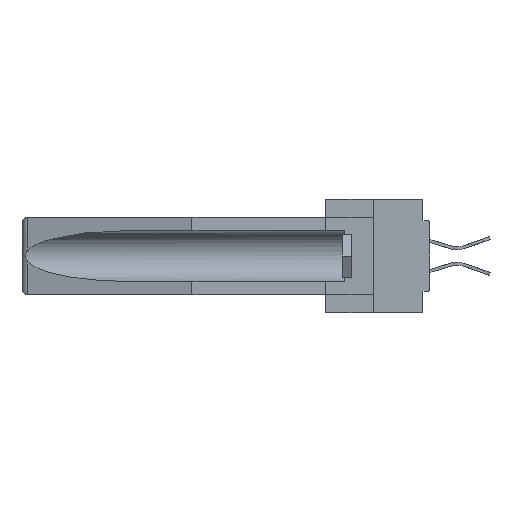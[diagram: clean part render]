
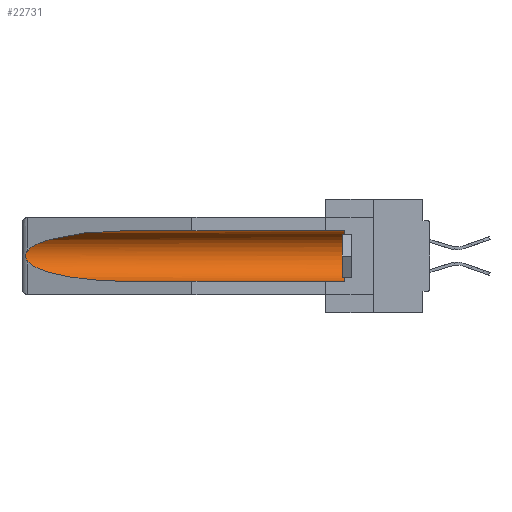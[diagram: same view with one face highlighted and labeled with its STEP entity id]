
A CAD part, left-side view. The second image highlights one B-rep face of the part: STEP entity #22731.
In plain terms, the highlighted cylindrical face has radius 2.857 mm (diameter 5.715 mm), a partial arc.
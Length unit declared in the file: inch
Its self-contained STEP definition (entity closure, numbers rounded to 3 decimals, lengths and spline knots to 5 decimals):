
#87 = DIRECTION ( 'NONE',  ( 0., 1., 0. ) ) ;
#772 = CARTESIAN_POINT ( 'NONE',  ( 0.155, 0.126, -0.1715 ) ) ;
#1857 =( BOUNDED_CURVE ( )  B_SPLINE_CURVE ( 3, ( #37850, #8240, #2736, #37587 ),
 .UNSPECIFIED., .F., .F. ) 
 B_SPLINE_CURVE_WITH_KNOTS ( ( 4, 4 ),
 ( 0.1948, 1.5708 ),
 .UNSPECIFIED. ) 
 CURVE ( )  GEOMETRIC_REPRESENTATION_ITEM ( )  RATIONAL_B_SPLINE_CURVE ( ( 1., 0.848, 0.848, 1. ) ) 
 REPRESENTATION_ITEM ( '' )  );
#2736 = CARTESIAN_POINT ( 'NONE',  ( 0.21114, 1.30732, -0.284 ) ) ;
#4269 = CARTESIAN_POINT ( 'NONE',  ( 0.26597, 1.5296, -0.19026 ) ) ;
#4793 = EDGE_CURVE ( 'NONE', #7415, #30920, #1857, .T. ) ;
#5750 = CARTESIAN_POINT ( 'NONE',  ( 0.155, -0.30754, -0.059 ) ) ;
#6039 = ORIENTED_EDGE ( 'NONE', *, *, #6914, .T. ) ;
#6296 = DIRECTION ( 'NONE',  ( 0., 1., 0. ) ) ;
#6306 = ORIENTED_EDGE ( 'NONE', *, *, #4793, .T. ) ;
#6914 = EDGE_CURVE ( 'NONE', #28909, #23332, #20168, .T. ) ;
#6995 = ORIENTED_EDGE ( 'NONE', *, *, #14055, .T. ) ;
#7080 = CARTESIAN_POINT ( 'NONE',  ( 0.2675, 1.53308, -0.17534 ) ) ;
#7415 = VERTEX_POINT ( 'NONE', #16191 ) ;
#8240 = CARTESIAN_POINT ( 'NONE',  ( 0.25451, 1.48313, -0.24835 ) ) ;
#8750 = CARTESIAN_POINT ( 'NONE',  ( 0.155, 1.07973, -0.284 ) ) ;
#9074 = CARTESIAN_POINT ( 'NONE',  ( 0.155, -0.30754, -0.284 ) ) ;
#9399 = CARTESIAN_POINT ( 'NONE',  ( 0.26654, 1.53092, -0.15636 ) ) ;
#10024 = CARTESIAN_POINT ( 'NONE',  ( 0.26537, 1.52718, -0.19328 ) ) ;
#10286 = FACE_OUTER_BOUND ( 'NONE', #32489, .T. ) ;
#10372 = CARTESIAN_POINT ( 'NONE',  ( 0.155, 1.07973, -0.059 ) ) ;
#10424 = CARTESIAN_POINT ( 'NONE',  ( 0.2673, 1.5327, -0.16383 ) ) ;
#10641 = CARTESIAN_POINT ( 'NONE',  ( 0.155, 1.07973, -0.059 ) ) ;
#11722 = AXIS2_PLACEMENT_3D ( 'NONE', #772, #21275, #12678 ) ;
#12678 = DIRECTION ( 'NONE',  ( 0., 0., 1. ) ) ;
#14055 = EDGE_CURVE ( 'NONE', #23332, #7415, #35924, .T. ) ;
#15910 = CARTESIAN_POINT ( 'NONE',  ( 0.26655, 1.53094, -0.18657 ) ) ;
#16191 = CARTESIAN_POINT ( 'NONE',  ( 0.26537, 1.52718, -0.19328 ) ) ;
#19042 = LINE ( 'NONE', #9074, #26849 ) ;
#19196 = CARTESIAN_POINT ( 'NONE',  ( 0.25451, 1.48313, -0.09465 ) ) ;
#19502 = EDGE_CURVE ( 'NONE', #28320, #19665, #35521, .T. ) ;
#19665 = VERTEX_POINT ( 'NONE', #27777 ) ;
#20168 =( BOUNDED_CURVE ( )  B_SPLINE_CURVE ( 3, ( #10372, #33806, #19196, #22140 ),
 .UNSPECIFIED., .F., .F. ) 
 B_SPLINE_CURVE_WITH_KNOTS ( ( 4, 4 ),
 ( 4.71239, 6.08839 ),
 .UNSPECIFIED. ) 
 CURVE ( )  GEOMETRIC_REPRESENTATION_ITEM ( )  RATIONAL_B_SPLINE_CURVE ( ( 1., 0.848, 0.848, 1. ) ) 
 REPRESENTATION_ITEM ( '' )  );
#21275 = DIRECTION ( 'NONE',  ( 0., -1., 0. ) ) ;
#22140 = CARTESIAN_POINT ( 'NONE',  ( 0.26537, 1.52718, -0.14972 ) ) ;
#22731 = ADVANCED_FACE ( 'NONE', ( #10286 ), #35518, .F. ) ;
#23332 = VERTEX_POINT ( 'NONE', #31109 ) ;
#23337 = ORIENTED_EDGE ( 'NONE', *, *, #19502, .T. ) ;
#23978 = CARTESIAN_POINT ( 'NONE',  ( 0.26597, 1.52961, -0.15275 ) ) ;
#26774 = CARTESIAN_POINT ( 'NONE',  ( 0.155, -0.30754, -0.1715 ) ) ;
#26849 = VECTOR ( 'NONE', #87, 39.37008 ) ;
#27563 = CARTESIAN_POINT ( 'NONE',  ( 0.2673, 1.53269, -0.17917 ) ) ;
#27777 = CARTESIAN_POINT ( 'NONE',  ( 0.155, 0.126, -0.059 ) ) ;
#28288 = CARTESIAN_POINT ( 'NONE',  ( 0.155, 0.126, -0.284 ) ) ;
#28320 = VERTEX_POINT ( 'NONE', #28288 ) ;
#28909 = VERTEX_POINT ( 'NONE', #10641 ) ;
#29865 = CARTESIAN_POINT ( 'NONE',  ( 0.2675, 1.53308, -0.16763 ) ) ;
#30920 = VERTEX_POINT ( 'NONE', #8750 ) ;
#31109 = CARTESIAN_POINT ( 'NONE',  ( 0.26537, 1.52718, -0.14972 ) ) ;
#31527 = EDGE_CURVE ( 'NONE', #19665, #28909, #34534, .T. ) ;
#32489 = EDGE_LOOP ( 'NONE', ( #6039, #6995, #6306, #33144, #23337, #37250 ) ) ;
#32511 = DIRECTION ( 'NONE',  ( 0., 1., 0. ) ) ;
#33144 = ORIENTED_EDGE ( 'NONE', *, *, #36436, .F. ) ;
#33579 = VECTOR ( 'NONE', #32511, 39.37008 ) ;
#33806 = CARTESIAN_POINT ( 'NONE',  ( 0.21114, 1.30732, -0.059 ) ) ;
#34534 = LINE ( 'NONE', #5750, #33579 ) ;
#35518 = CYLINDRICAL_SURFACE ( 'NONE', #35853, 0.1125 ) ;
#35521 = CIRCLE ( 'NONE', #11722, 0.1125 ) ;
#35853 = AXIS2_PLACEMENT_3D ( 'NONE', #26774, #6296, #35863 ) ;
#35863 = DIRECTION ( 'NONE',  ( 0., 0., 1. ) ) ;
#35924 = B_SPLINE_CURVE_WITH_KNOTS ( 'NONE', 3,
 ( #36421, #23978, #9399, #10424, #29865, #7080, #27563, #15910, #4269, #10024 ),
 .UNSPECIFIED., .F., .F.,
 ( 4, 2, 2, 2, 4 ),
 ( 0., 0.00029, 0.00058, 0.00087, 0.00117 ),
 .UNSPECIFIED. ) ;
#36421 = CARTESIAN_POINT ( 'NONE',  ( 0.26537, 1.52718, -0.14972 ) ) ;
#36436 = EDGE_CURVE ( 'NONE', #28320, #30920, #19042, .T. ) ;
#37250 = ORIENTED_EDGE ( 'NONE', *, *, #31527, .T. ) ;
#37587 = CARTESIAN_POINT ( 'NONE',  ( 0.155, 1.07973, -0.284 ) ) ;
#37850 = CARTESIAN_POINT ( 'NONE',  ( 0.26537, 1.52718, -0.19328 ) ) ;
